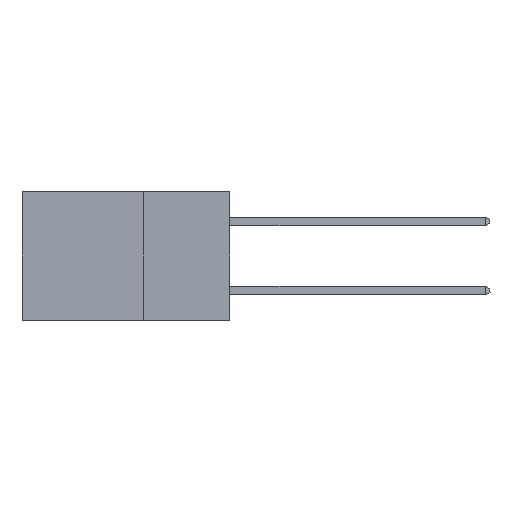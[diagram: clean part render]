
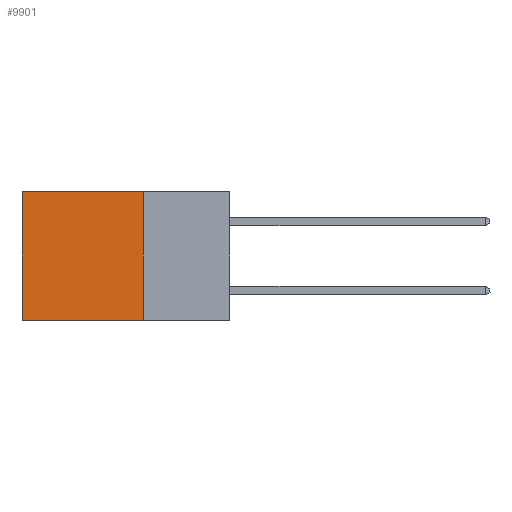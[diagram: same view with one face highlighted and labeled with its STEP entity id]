
A CAD part, left-side view. The second image highlights one B-rep face of the part: STEP entity #9901.
In plain terms, the highlighted planar face has unit normal (-1, 0, 0).
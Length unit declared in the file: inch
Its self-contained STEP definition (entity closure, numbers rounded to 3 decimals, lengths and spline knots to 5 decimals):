
#142 = AXIS2_PLACEMENT_3D ( 'NONE', #6157, #15659, #1964 ) ;
#1295 = VERTEX_POINT ( 'NONE', #12255 ) ;
#1362 = CARTESIAN_POINT ( 'NONE',  ( 0.298, 0.25, 0. ) ) ;
#1964 = DIRECTION ( 'NONE',  ( 0., 0., -1. ) ) ;
#2064 = DIRECTION ( 'NONE',  ( 0., 1., 0. ) ) ;
#2065 = VERTEX_POINT ( 'NONE', #6879 ) ;
#3080 = LINE ( 'NONE', #1362, #16409 ) ;
#3444 = DIRECTION ( 'NONE',  ( 0., 1., 0. ) ) ;
#3659 = VECTOR ( 'NONE', #2064, 39.37008 ) ;
#3877 = LINE ( 'NONE', #8866, #3659 ) ;
#4148 = VERTEX_POINT ( 'NONE', #7851 ) ;
#6157 = CARTESIAN_POINT ( 'NONE',  ( 0.298, 0.25, 0. ) ) ;
#6879 = CARTESIAN_POINT ( 'NONE',  ( 0.298, 0.6, -0.37 ) ) ;
#7815 = EDGE_CURVE ( 'NONE', #9784, #2065, #8578, .T. ) ;
#7851 = CARTESIAN_POINT ( 'NONE',  ( 0.298, 0.25, -0.37 ) ) ;
#8578 = LINE ( 'NONE', #9229, #17228 ) ;
#8866 = CARTESIAN_POINT ( 'NONE',  ( 0.298, 0.25, 0. ) ) ;
#9229 = CARTESIAN_POINT ( 'NONE',  ( 0.298, 0.6, 0. ) ) ;
#9436 = EDGE_CURVE ( 'NONE', #1295, #9784, #3877, .T. ) ;
#9784 = VERTEX_POINT ( 'NONE', #13368 ) ;
#9901 = ADVANCED_FACE ( 'NONE', ( #15035 ), #14180, .F. ) ;
#10564 = DIRECTION ( 'NONE',  ( 0., 0., -1. ) ) ;
#11597 = EDGE_LOOP ( 'NONE', ( #13195, #14841, #16711, #15651 ) ) ;
#12255 = CARTESIAN_POINT ( 'NONE',  ( 0.298, 0.25, 0. ) ) ;
#13084 = EDGE_CURVE ( 'NONE', #1295, #4148, #3080, .T. ) ;
#13195 = ORIENTED_EDGE ( 'NONE', *, *, #7815, .T. ) ;
#13368 = CARTESIAN_POINT ( 'NONE',  ( 0.298, 0.6, 0. ) ) ;
#13540 = EDGE_CURVE ( 'NONE', #4148, #2065, #13838, .T. ) ;
#13838 = LINE ( 'NONE', #16997, #14067 ) ;
#14067 = VECTOR ( 'NONE', #3444, 39.37008 ) ;
#14180 = PLANE ( 'NONE',  #142 ) ;
#14841 = ORIENTED_EDGE ( 'NONE', *, *, #13540, .F. ) ;
#15035 = FACE_OUTER_BOUND ( 'NONE', #11597, .T. ) ;
#15651 = ORIENTED_EDGE ( 'NONE', *, *, #9436, .T. ) ;
#15659 = DIRECTION ( 'NONE',  ( 1., 0., 0. ) ) ;
#16137 = DIRECTION ( 'NONE',  ( 0., 0., -1. ) ) ;
#16409 = VECTOR ( 'NONE', #16137, 39.37008 ) ;
#16711 = ORIENTED_EDGE ( 'NONE', *, *, #13084, .F. ) ;
#16997 = CARTESIAN_POINT ( 'NONE',  ( 0.298, 0.25, -0.37 ) ) ;
#17228 = VECTOR ( 'NONE', #10564, 39.37008 ) ;
